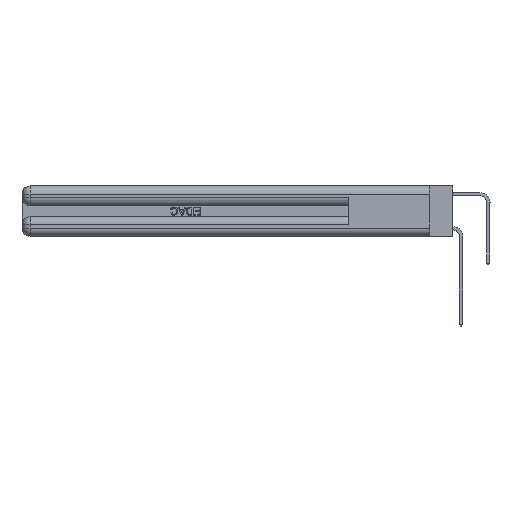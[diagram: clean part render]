
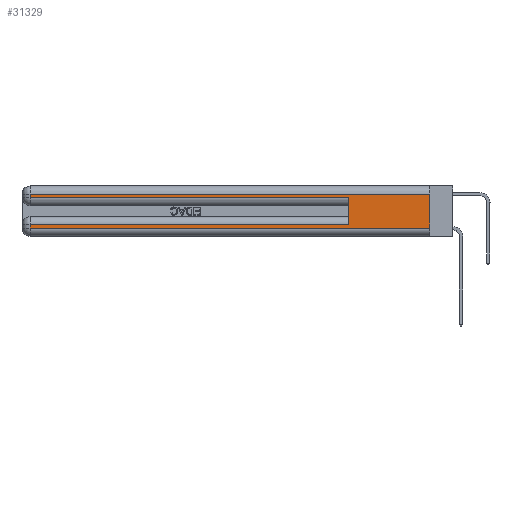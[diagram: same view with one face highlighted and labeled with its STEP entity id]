
A CAD part, left-side view. The second image highlights one B-rep face of the part: STEP entity #31329.
In plain terms, the highlighted planar face has unit normal (-1, 0, 0).
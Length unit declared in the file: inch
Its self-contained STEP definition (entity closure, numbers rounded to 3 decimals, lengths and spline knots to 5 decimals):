
#126 = VECTOR ( 'NONE', #33337, 39.37008 ) ;
#255 = CARTESIAN_POINT ( 'NONE',  ( 0., 2.94, 0.37 ) ) ;
#266 = ORIENTED_EDGE ( 'NONE', *, *, #6339, .T. ) ;
#357 = EDGE_LOOP ( 'NONE', ( #7493, #6195, #3179, #266, #31188, #3273, #9941, #34861 ) ) ;
#1279 = EDGE_CURVE ( 'NONE', #35974, #35071, #11831, .T. ) ;
#2256 = CARTESIAN_POINT ( 'NONE',  ( 0., 0., 0.31 ) ) ;
#3179 = ORIENTED_EDGE ( 'NONE', *, *, #27033, .T. ) ;
#3273 = ORIENTED_EDGE ( 'NONE', *, *, #1279, .T. ) ;
#3848 = VECTOR ( 'NONE', #29946, 39.37008 ) ;
#4240 = CARTESIAN_POINT ( 'NONE',  ( 0., 2.94, 0.085 ) ) ;
#4954 = LINE ( 'NONE', #30413, #20762 ) ;
#5887 = LINE ( 'NONE', #15994, #31137 ) ;
#6195 = ORIENTED_EDGE ( 'NONE', *, *, #34086, .T. ) ;
#6225 = CARTESIAN_POINT ( 'NONE',  ( 0., 0.6, 0.085 ) ) ;
#6339 = EDGE_CURVE ( 'NONE', #33354, #6823, #22660, .T. ) ;
#6823 = VERTEX_POINT ( 'NONE', #12876 ) ;
#7436 = DIRECTION ( 'NONE',  ( 0., 0., -1. ) ) ;
#7493 = ORIENTED_EDGE ( 'NONE', *, *, #33234, .F. ) ;
#9748 = DIRECTION ( 'NONE',  ( 0., 0., 1. ) ) ;
#9941 = ORIENTED_EDGE ( 'NONE', *, *, #22578, .T. ) ;
#10970 = VECTOR ( 'NONE', #34818, 39.37008 ) ;
#11318 = AXIS2_PLACEMENT_3D ( 'NONE', #27474, #36592, #27736 ) ;
#11831 = LINE ( 'NONE', #35795, #3848 ) ;
#12876 = CARTESIAN_POINT ( 'NONE',  ( 0., 0.6, 0.285 ) ) ;
#13183 = EDGE_CURVE ( 'NONE', #35974, #6823, #4954, .T. ) ;
#13280 = DIRECTION ( 'NONE',  ( 0., -1., 0. ) ) ;
#13310 = CARTESIAN_POINT ( 'NONE',  ( 0., 2.94, 0.37 ) ) ;
#13543 = CARTESIAN_POINT ( 'NONE',  ( 0., 2.94, 0.285 ) ) ;
#14499 = CARTESIAN_POINT ( 'NONE',  ( 0., 2.94, 0.06 ) ) ;
#15833 = CARTESIAN_POINT ( 'NONE',  ( 0., 2.94, 0.31 ) ) ;
#15994 = CARTESIAN_POINT ( 'NONE',  ( 0., 0., 0.37 ) ) ;
#18479 = VECTOR ( 'NONE', #13280, 39.37008 ) ;
#18817 = DIRECTION ( 'NONE',  ( 0., -1., 0. ) ) ;
#20685 = LINE ( 'NONE', #255, #126 ) ;
#20762 = VECTOR ( 'NONE', #9748, 39.37008 ) ;
#22247 = CARTESIAN_POINT ( 'NONE',  ( 0., 0., 0.06 ) ) ;
#22578 = EDGE_CURVE ( 'NONE', #35071, #34643, #20685, .T. ) ;
#22660 = LINE ( 'NONE', #24358, #31602 ) ;
#23268 = VECTOR ( 'NONE', #7436, 39.37008 ) ;
#24358 = CARTESIAN_POINT ( 'NONE',  ( 0., 0., 0.285 ) ) ;
#24587 = PLANE ( 'NONE',  #11318 ) ;
#26229 = CARTESIAN_POINT ( 'NONE',  ( 0., 0., 0.06 ) ) ;
#26842 = LINE ( 'NONE', #2256, #10970 ) ;
#27033 = EDGE_CURVE ( 'NONE', #37204, #33354, #31230, .T. ) ;
#27474 = CARTESIAN_POINT ( 'NONE',  ( 0., 0., 0.37 ) ) ;
#27736 = DIRECTION ( 'NONE',  ( 0., 0., -1. ) ) ;
#28562 = CARTESIAN_POINT ( 'NONE',  ( 0., 0., 0.31 ) ) ;
#29946 = DIRECTION ( 'NONE',  ( 0., 1., 0. ) ) ;
#30413 = CARTESIAN_POINT ( 'NONE',  ( 0., 0.6, 0.145 ) ) ;
#30609 = VERTEX_POINT ( 'NONE', #26229 ) ;
#30792 = FACE_OUTER_BOUND ( 'NONE', #357, .T. ) ;
#31137 = VECTOR ( 'NONE', #33928, 39.37008 ) ;
#31139 = VERTEX_POINT ( 'NONE', #28562 ) ;
#31188 = ORIENTED_EDGE ( 'NONE', *, *, #13183, .F. ) ;
#31230 = LINE ( 'NONE', #13310, #23268 ) ;
#31329 = ADVANCED_FACE ( 'NONE', ( #30792 ), #24587, .F. ) ;
#31602 = VECTOR ( 'NONE', #18817, 39.37008 ) ;
#33234 = EDGE_CURVE ( 'NONE', #31139, #30609, #5887, .T. ) ;
#33337 = DIRECTION ( 'NONE',  ( 0., 0., -1. ) ) ;
#33354 = VERTEX_POINT ( 'NONE', #13543 ) ;
#33928 = DIRECTION ( 'NONE',  ( 0., 0., -1. ) ) ;
#34086 = EDGE_CURVE ( 'NONE', #31139, #37204, #26842, .T. ) ;
#34643 = VERTEX_POINT ( 'NONE', #14499 ) ;
#34818 = DIRECTION ( 'NONE',  ( 0., 1., 0. ) ) ;
#34861 = ORIENTED_EDGE ( 'NONE', *, *, #36615, .T. ) ;
#34957 = LINE ( 'NONE', #22247, #18479 ) ;
#35071 = VERTEX_POINT ( 'NONE', #4240 ) ;
#35795 = CARTESIAN_POINT ( 'NONE',  ( 0., 0., 0.085 ) ) ;
#35974 = VERTEX_POINT ( 'NONE', #6225 ) ;
#36592 = DIRECTION ( 'NONE',  ( 1., 0., 0. ) ) ;
#36615 = EDGE_CURVE ( 'NONE', #34643, #30609, #34957, .T. ) ;
#37204 = VERTEX_POINT ( 'NONE', #15833 ) ;
